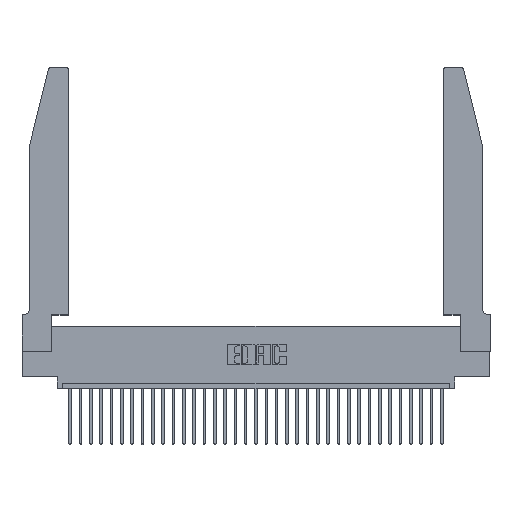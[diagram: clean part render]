
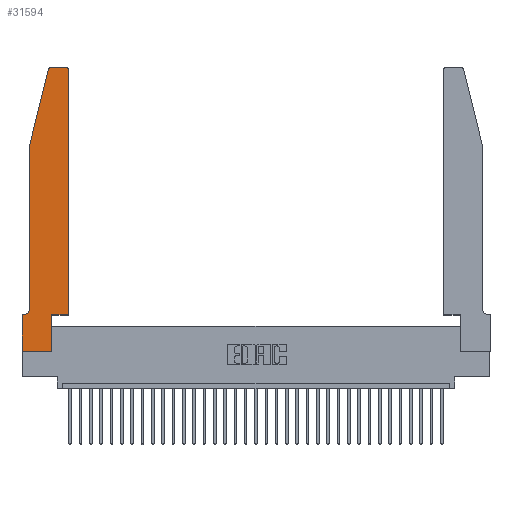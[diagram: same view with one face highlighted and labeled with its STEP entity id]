
A CAD part, top view. The second image highlights one B-rep face of the part: STEP entity #31594.
In plain terms, the highlighted planar face has unit normal (0, 0, 1).
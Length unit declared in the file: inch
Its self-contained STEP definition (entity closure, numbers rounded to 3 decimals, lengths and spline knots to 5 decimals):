
#554 = CARTESIAN_POINT ( 'NONE',  ( 0.284, 2.75, 0.37 ) ) ;
#701 = CARTESIAN_POINT ( 'NONE',  ( 0.25487, 2.72718, 0.37 ) ) ;
#761 = VECTOR ( 'NONE', #24265, 39.37008 ) ;
#883 = DIRECTION ( 'NONE',  ( 0., 0., -1. ) ) ;
#1164 = EDGE_CURVE ( 'NONE', #15190, #5946, #7179, .T. ) ;
#1177 = DIRECTION ( 'NONE',  ( 1., 0., 0. ) ) ;
#1386 = CARTESIAN_POINT ( 'NONE',  ( 0., 0.35, 0.37 ) ) ;
#1483 = VECTOR ( 'NONE', #19601, 39.37008 ) ;
#1817 = CARTESIAN_POINT ( 'NONE',  ( 0.284, 2.72, 0.37 ) ) ;
#1942 = ORIENTED_EDGE ( 'NONE', *, *, #2213, .T. ) ;
#2057 = LINE ( 'NONE', #23500, #24292 ) ;
#2213 = EDGE_CURVE ( 'NONE', #31261, #30258, #21262, .T. ) ;
#2312 = DIRECTION ( 'NONE',  ( 1., 0., 0. ) ) ;
#2991 = CIRCLE ( 'NONE', #14309, 0.03 ) ;
#3088 = ORIENTED_EDGE ( 'NONE', *, *, #22761, .T. ) ;
#3871 = ORIENTED_EDGE ( 'NONE', *, *, #10085, .T. ) ;
#4031 = CARTESIAN_POINT ( 'NONE',  ( 0.4505, 0.35, 0.37 ) ) ;
#4066 = VECTOR ( 'NONE', #28126, 39.37008 ) ;
#4108 = LINE ( 'NONE', #31468, #33197 ) ;
#4129 = CIRCLE ( 'NONE', #6225, 0.07 ) ;
#4311 = EDGE_CURVE ( 'NONE', #30258, #9381, #4539, .T. ) ;
#4529 = DIRECTION ( 'NONE',  ( 0., -1., 0. ) ) ;
#4539 = LINE ( 'NONE', #29161, #15869 ) ;
#4661 = LINE ( 'NONE', #25795, #26880 ) ;
#4779 = CARTESIAN_POINT ( 'NONE',  ( 0.2865, 0., 0.37 ) ) ;
#4965 = AXIS2_PLACEMENT_3D ( 'NONE', #1386, #21576, #1177 ) ;
#5474 = DIRECTION ( 'NONE',  ( 0., -1., 0. ) ) ;
#5717 = CARTESIAN_POINT ( 'NONE',  ( 0.0055, 0.42, 0.37 ) ) ;
#5946 = VERTEX_POINT ( 'NONE', #33403 ) ;
#6225 = AXIS2_PLACEMENT_3D ( 'NONE', #5717, #883, #23755 ) ;
#6705 = DIRECTION ( 'NONE',  ( 0., 0., 1. ) ) ;
#7179 = LINE ( 'NONE', #19086, #761 ) ;
#7514 = CARTESIAN_POINT ( 'NONE',  ( 0.2605, 2.75, 0.37 ) ) ;
#9219 = ORIENTED_EDGE ( 'NONE', *, *, #4311, .T. ) ;
#9344 = EDGE_CURVE ( 'NONE', #9451, #15190, #4129, .T. ) ;
#9381 = VERTEX_POINT ( 'NONE', #10801 ) ;
#9451 = VERTEX_POINT ( 'NONE', #23871 ) ;
#9594 = VERTEX_POINT ( 'NONE', #27614 ) ;
#9799 = ORIENTED_EDGE ( 'NONE', *, *, #24410, .T. ) ;
#10085 = EDGE_CURVE ( 'NONE', #9594, #23293, #23865, .T. ) ;
#10781 = ORIENTED_EDGE ( 'NONE', *, *, #13455, .T. ) ;
#10801 = CARTESIAN_POINT ( 'NONE',  ( 0.4505, 0.35, 0.37 ) ) ;
#11422 = PLANE ( 'NONE',  #4965 ) ;
#11485 = DIRECTION ( 'NONE',  ( 1., 0., 0. ) ) ;
#11678 = CARTESIAN_POINT ( 'NONE',  ( 0.2865, 0.35, 0.37 ) ) ;
#11963 = CARTESIAN_POINT ( 'NONE',  ( 0.0755, 2., 0.37 ) ) ;
#12637 = CARTESIAN_POINT ( 'NONE',  ( 0., 0., 0.37 ) ) ;
#13227 = LINE ( 'NONE', #4031, #1483 ) ;
#13237 = VERTEX_POINT ( 'NONE', #701 ) ;
#13376 = DIRECTION ( 'NONE',  ( 0., 1., 0. ) ) ;
#13455 = EDGE_CURVE ( 'NONE', #9381, #17936, #13227, .T. ) ;
#13686 = DIRECTION ( 'NONE',  ( -0.239, -0.971, 0. ) ) ;
#13708 = EDGE_CURVE ( 'NONE', #15253, #31261, #4661, .T. ) ;
#13896 = CIRCLE ( 'NONE', #18993, 0.03 ) ;
#14309 = AXIS2_PLACEMENT_3D ( 'NONE', #26899, #6705, #19344 ) ;
#14831 = ORIENTED_EDGE ( 'NONE', *, *, #30459, .T. ) ;
#15146 = VERTEX_POINT ( 'NONE', #11963 ) ;
#15190 = VERTEX_POINT ( 'NONE', #32599 ) ;
#15253 = VERTEX_POINT ( 'NONE', #12637 ) ;
#15583 = DIRECTION ( 'NONE',  ( 1., 0., 0. ) ) ;
#15869 = VECTOR ( 'NONE', #11485, 39.37008 ) ;
#15980 = ORIENTED_EDGE ( 'NONE', *, *, #26361, .T. ) ;
#17936 = VERTEX_POINT ( 'NONE', #25772 ) ;
#18605 = LINE ( 'NONE', #30338, #28693 ) ;
#18904 = FACE_OUTER_BOUND ( 'NONE', #23943, .T. ) ;
#18993 = AXIS2_PLACEMENT_3D ( 'NONE', #1817, #25624, #15583 ) ;
#19007 = ORIENTED_EDGE ( 'NONE', *, *, #9344, .T. ) ;
#19086 = CARTESIAN_POINT ( 'NONE',  ( 0.0755, 0.35, 0.37 ) ) ;
#19344 = DIRECTION ( 'NONE',  ( 1., 0., 0. ) ) ;
#19601 = DIRECTION ( 'NONE',  ( 0., 1., 0. ) ) ;
#21262 = LINE ( 'NONE', #28776, #32939 ) ;
#21576 = DIRECTION ( 'NONE',  ( 0., 0., 1. ) ) ;
#22761 = EDGE_CURVE ( 'NONE', #17936, #9594, #2991, .T. ) ;
#23293 = VERTEX_POINT ( 'NONE', #554 ) ;
#23328 = ORIENTED_EDGE ( 'NONE', *, *, #1164, .T. ) ;
#23500 = CARTESIAN_POINT ( 'NONE',  ( 0.0755, 2., 0.37 ) ) ;
#23755 = DIRECTION ( 'NONE',  ( -1., 0., 0. ) ) ;
#23856 = EDGE_CURVE ( 'NONE', #13237, #15146, #4108, .T. ) ;
#23865 = LINE ( 'NONE', #7514, #4066 ) ;
#23871 = CARTESIAN_POINT ( 'NONE',  ( 0.0755, 0.42, 0.37 ) ) ;
#23943 = EDGE_LOOP ( 'NONE', ( #3871, #14831, #30730, #9799, #19007, #23328, #15980, #30997, #1942, #9219, #10781, #3088 ) ) ;
#24265 = DIRECTION ( 'NONE',  ( -1., 0., 0. ) ) ;
#24292 = VECTOR ( 'NONE', #5474, 39.37008 ) ;
#24410 = EDGE_CURVE ( 'NONE', #15146, #9451, #2057, .T. ) ;
#25624 = DIRECTION ( 'NONE',  ( 0., 0., 1. ) ) ;
#25772 = CARTESIAN_POINT ( 'NONE',  ( 0.4505, 2.72, 0.37 ) ) ;
#25795 = CARTESIAN_POINT ( 'NONE',  ( 0., 0., 0.37 ) ) ;
#26361 = EDGE_CURVE ( 'NONE', #5946, #15253, #18605, .T. ) ;
#26880 = VECTOR ( 'NONE', #2312, 39.37008 ) ;
#26899 = CARTESIAN_POINT ( 'NONE',  ( 0.4205, 2.72, 0.37 ) ) ;
#27614 = CARTESIAN_POINT ( 'NONE',  ( 0.4205, 2.75, 0.37 ) ) ;
#28126 = DIRECTION ( 'NONE',  ( -1., 0., 0. ) ) ;
#28693 = VECTOR ( 'NONE', #4529, 39.37008 ) ;
#28776 = CARTESIAN_POINT ( 'NONE',  ( 0.2865, 0.35, 0.37 ) ) ;
#29161 = CARTESIAN_POINT ( 'NONE',  ( 0.4505, 0.35, 0.37 ) ) ;
#30258 = VERTEX_POINT ( 'NONE', #11678 ) ;
#30338 = CARTESIAN_POINT ( 'NONE',  ( 0., 0., 0.37 ) ) ;
#30459 = EDGE_CURVE ( 'NONE', #23293, #13237, #13896, .T. ) ;
#30730 = ORIENTED_EDGE ( 'NONE', *, *, #23856, .T. ) ;
#30997 = ORIENTED_EDGE ( 'NONE', *, *, #13708, .T. ) ;
#31261 = VERTEX_POINT ( 'NONE', #4779 ) ;
#31468 = CARTESIAN_POINT ( 'NONE',  ( 0.0755, 2., 0.37 ) ) ;
#31594 = ADVANCED_FACE ( 'NONE', ( #18904 ), #11422, .T. ) ;
#32599 = CARTESIAN_POINT ( 'NONE',  ( 0.0055, 0.35, 0.37 ) ) ;
#32939 = VECTOR ( 'NONE', #13376, 39.37008 ) ;
#33197 = VECTOR ( 'NONE', #13686, 39.37008 ) ;
#33403 = CARTESIAN_POINT ( 'NONE',  ( 0., 0.35, 0.37 ) ) ;
